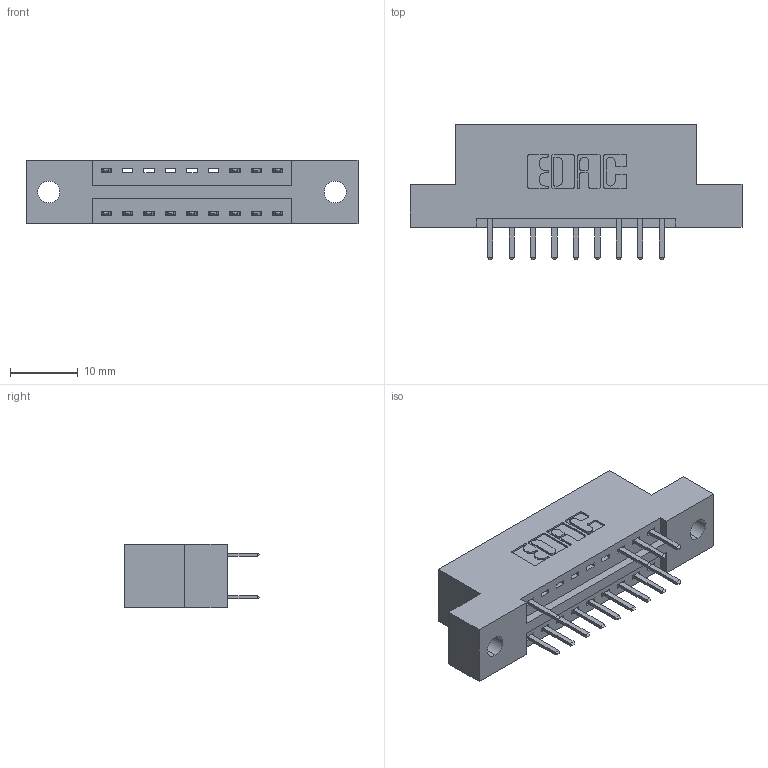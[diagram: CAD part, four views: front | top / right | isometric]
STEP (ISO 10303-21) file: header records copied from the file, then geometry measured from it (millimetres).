
FILE_DESCRIPTION (( 'STEP AP203' ), '1' );
FILE_NAME ('346-018-520-202.STEP', '2018-08-20T07:01:34', ( '' ), ( '' ), 'SwSTEP 2.0', 'SolidWorks 2016', '' );
FILE_SCHEMA (( 'CONFIG_CONTROL_DESIGN' ));
Length unit declared in the file: inch
Products named in the file (3): 346 Part_Flush Mounting Lugs - 0.128 Dia; 345-292-001_345-293-120; 346-018-520-202
Assembly tree (14 placements, depth 2):
  346-018-520-202
    346 Part_Flush Mounting Lugs - 0.128 Dia
    345-292-001_345-293-120  x13
Bounding box: 49.15 x 20.02 x 9.4 mm (x, y, z)
Volume: 4448.9 mm3; surface area: 5054.6 mm2
Topology: 14 solids, 14 shells, 880 faces, 2553 edges, 1666 vertices
Faces by surface type: plane 582, cylinder 298
Entity records: 10273 total; most frequent: CARTESIAN_POINT 1771, ORIENTED_EDGE 1698, DIRECTION 1595, EDGE_CURVE 849, VECTOR 677, LINE 677, VERTEX_POINT 562, AXIS2_PLACEMENT_3D 459
